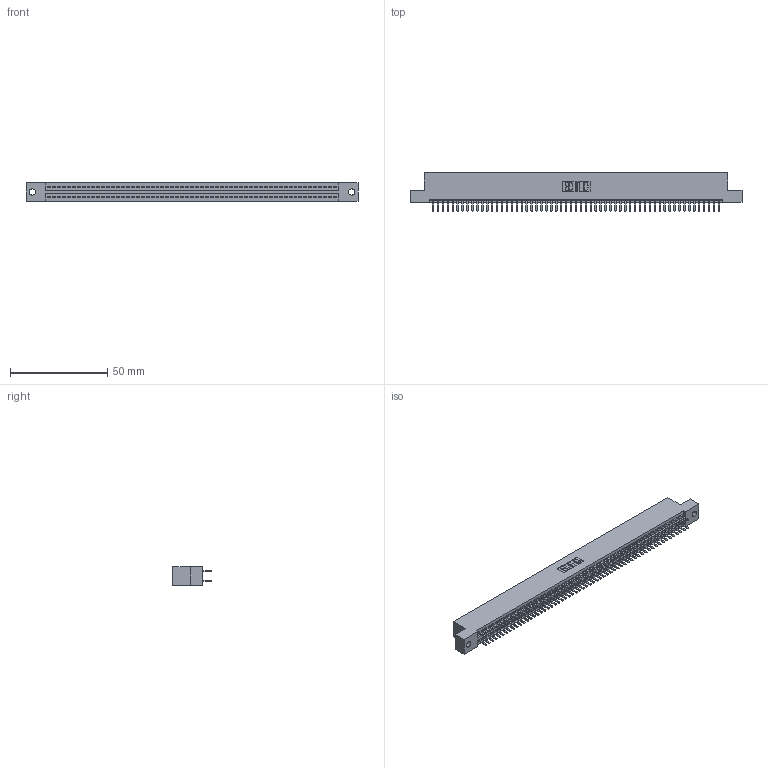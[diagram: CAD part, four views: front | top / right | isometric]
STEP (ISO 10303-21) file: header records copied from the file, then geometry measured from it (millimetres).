
FILE_DESCRIPTION (( 'STEP AP203' ), '1' );
FILE_NAME ('345-118-520-202.STEP', '2019-11-05T18:16:00', ( '' ), ( '' ), 'SwSTEP 2.0', 'SolidWorks 2016', '' );
FILE_SCHEMA (( 'CONFIG_CONTROL_DESIGN' ));
Length unit declared in the file: inch
Products named in the file (3): 345-292-001_345-293-120; 345-118-520-202; 345 Part_Flush Mounting Lugs - 0.128 Dia
Assembly tree (119 placements, depth 2):
  345-118-520-202
    345 Part_Flush Mounting Lugs - 0.128 Dia
    345-292-001_345-293-120  x118
Bounding box: 171.07 x 19.68 x 9.4 mm (x, y, z)
Volume: 16687.1 mm3; surface area: 24612.5 mm2
Topology: 119 solids, 119 shells, 6498 faces, 18867 edges, 12262 vertices
Faces by surface type: plane 4210, cylinder 2288
Entity records: 44121 total; most frequent: CARTESIAN_POINT 7392, ORIENTED_EDGE 7314, DIRECTION 6485, EDGE_CURVE 3657, LINE 3285, VECTOR 3285, VERTEX_POINT 2434, AXIS2_PLACEMENT_3D 1600
